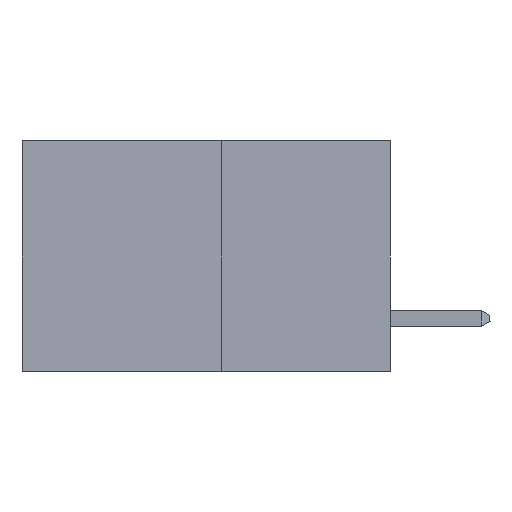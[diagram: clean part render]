
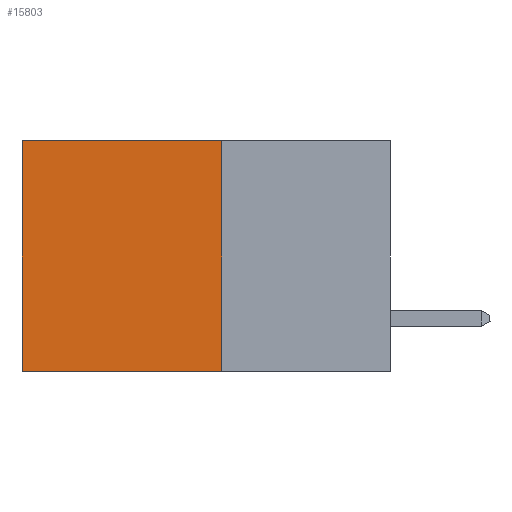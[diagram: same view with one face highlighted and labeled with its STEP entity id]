
A CAD part, left-side view. The second image highlights one B-rep face of the part: STEP entity #15803.
In plain terms, the highlighted planar face has unit normal (-1, 0, 0).
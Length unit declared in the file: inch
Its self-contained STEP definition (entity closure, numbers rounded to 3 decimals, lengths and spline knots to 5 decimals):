
#1243 = LINE ( 'NONE', #5101, #19285 ) ;
#1646 = DIRECTION ( 'NONE',  ( 1., 0., 0. ) ) ;
#1658 = DIRECTION ( 'NONE',  ( 0., 1., 0. ) ) ;
#1682 = LINE ( 'NONE', #22443, #10791 ) ;
#2856 = VERTEX_POINT ( 'NONE', #15247 ) ;
#3041 = VERTEX_POINT ( 'NONE', #4287 ) ;
#3752 = EDGE_LOOP ( 'NONE', ( #6271, #5897, #6537, #12119 ) ) ;
#4287 = CARTESIAN_POINT ( 'NONE',  ( 0.277, 0.27, 0. ) ) ;
#5101 = CARTESIAN_POINT ( 'NONE',  ( 0.277, 0.59, -0.37 ) ) ;
#5825 = VECTOR ( 'NONE', #13341, 39.37008 ) ;
#5897 = ORIENTED_EDGE ( 'NONE', *, *, #12086, .F. ) ;
#6271 = ORIENTED_EDGE ( 'NONE', *, *, #19859, .T. ) ;
#6537 = ORIENTED_EDGE ( 'NONE', *, *, #20901, .F. ) ;
#9520 = FACE_OUTER_BOUND ( 'NONE', #3752, .T. ) ;
#9522 = VECTOR ( 'NONE', #1658, 39.37008 ) ;
#10711 = PLANE ( 'NONE',  #17561 ) ;
#10791 = VECTOR ( 'NONE', #13693, 39.37008 ) ;
#10949 = EDGE_CURVE ( 'NONE', #3041, #22091, #14349, .T. ) ;
#11513 = CARTESIAN_POINT ( 'NONE',  ( 0.277, 0.27, -0.37 ) ) ;
#12086 = EDGE_CURVE ( 'NONE', #13429, #2856, #1682, .T. ) ;
#12119 = ORIENTED_EDGE ( 'NONE', *, *, #10949, .T. ) ;
#12544 = CARTESIAN_POINT ( 'NONE',  ( 0.277, 0.27, -0.37 ) ) ;
#13341 = DIRECTION ( 'NONE',  ( 0., 0., -1. ) ) ;
#13429 = VERTEX_POINT ( 'NONE', #15363 ) ;
#13693 = DIRECTION ( 'NONE',  ( 0., 1., 0. ) ) ;
#14349 = LINE ( 'NONE', #19610, #9522 ) ;
#14377 = DIRECTION ( 'NONE',  ( 0., 0., -1. ) ) ;
#15247 = CARTESIAN_POINT ( 'NONE',  ( 0.277, 0.59, -0.37 ) ) ;
#15363 = CARTESIAN_POINT ( 'NONE',  ( 0.277, 0.27, -0.37 ) ) ;
#15803 = ADVANCED_FACE ( 'NONE', ( #9520 ), #10711, .F. ) ;
#17561 = AXIS2_PLACEMENT_3D ( 'NONE', #12544, #1646, #14377 ) ;
#18657 = CARTESIAN_POINT ( 'NONE',  ( 0.277, 0.59, 0. ) ) ;
#19285 = VECTOR ( 'NONE', #19421, 39.37008 ) ;
#19421 = DIRECTION ( 'NONE',  ( 0., 0., -1. ) ) ;
#19610 = CARTESIAN_POINT ( 'NONE',  ( 0.277, 0.27, 0. ) ) ;
#19859 = EDGE_CURVE ( 'NONE', #22091, #2856, #1243, .T. ) ;
#20077 = LINE ( 'NONE', #11513, #5825 ) ;
#20901 = EDGE_CURVE ( 'NONE', #3041, #13429, #20077, .T. ) ;
#22091 = VERTEX_POINT ( 'NONE', #18657 ) ;
#22443 = CARTESIAN_POINT ( 'NONE',  ( 0.277, 0.27, -0.37 ) ) ;
